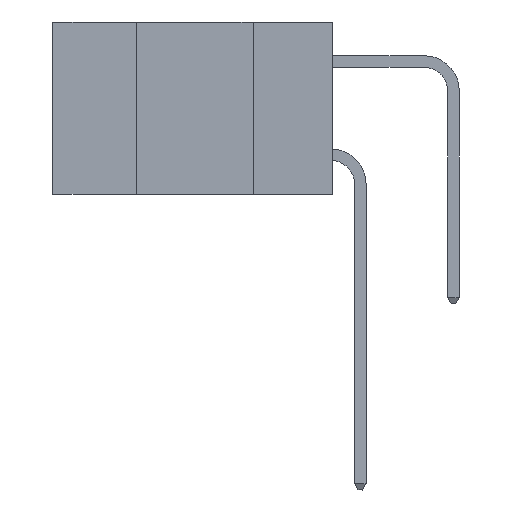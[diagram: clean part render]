
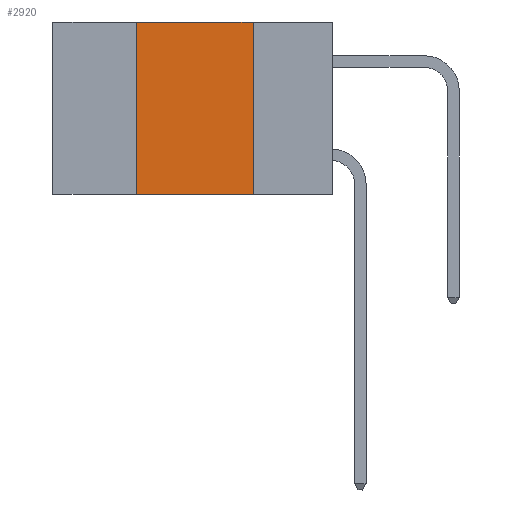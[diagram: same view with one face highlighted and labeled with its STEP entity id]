
A CAD part, left-side view. The second image highlights one B-rep face of the part: STEP entity #2920.
In plain terms, the highlighted planar face has unit normal (-1, 0, 0).
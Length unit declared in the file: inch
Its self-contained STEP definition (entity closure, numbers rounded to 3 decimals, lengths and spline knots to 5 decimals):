
#825 = EDGE_CURVE ( 'NONE', #7710, #1004, #13424, .T. ) ;
#835 = DIRECTION ( 'NONE',  ( 0., -1., 0. ) ) ;
#1004 = VERTEX_POINT ( 'NONE', #12930 ) ;
#1576 = VERTEX_POINT ( 'NONE', #9595 ) ;
#1838 = EDGE_LOOP ( 'NONE', ( #1877, #1987, #2013, #2182 ) ) ;
#1877 = ORIENTED_EDGE ( 'NONE', *, *, #9622, .F. ) ;
#1918 = VECTOR ( 'NONE', #5620, 39.37008 ) ;
#1955 = VERTEX_POINT ( 'NONE', #13369 ) ;
#1987 = ORIENTED_EDGE ( 'NONE', *, *, #13749, .F. ) ;
#2013 = ORIENTED_EDGE ( 'NONE', *, *, #4867, .F. ) ;
#2172 = FACE_OUTER_BOUND ( 'NONE', #1838, .T. ) ;
#2182 = ORIENTED_EDGE ( 'NONE', *, *, #825, .T. ) ;
#2338 = CARTESIAN_POINT ( 'NONE',  ( 0., 0.6, 0. ) ) ;
#2412 = LINE ( 'NONE', #2338, #13441 ) ;
#2836 = CARTESIAN_POINT ( 'NONE',  ( 0., 0.42, -0.37 ) ) ;
#2920 = ADVANCED_FACE ( 'NONE', ( #2172 ), #12034, .F. ) ;
#4664 = DIRECTION ( 'NONE',  ( 0., -1., 0. ) ) ;
#4845 = CARTESIAN_POINT ( 'NONE',  ( 0., 0.42, 0. ) ) ;
#4867 = EDGE_CURVE ( 'NONE', #7710, #1955, #12949, .T. ) ;
#5620 = DIRECTION ( 'NONE',  ( 0., 0., 1. ) ) ;
#5659 = CARTESIAN_POINT ( 'NONE',  ( 0., 0.6, -0.37 ) ) ;
#6917 = AXIS2_PLACEMENT_3D ( 'NONE', #8811, #9266, #10888 ) ;
#7131 = CARTESIAN_POINT ( 'NONE',  ( 0., 0.17, 0. ) ) ;
#7147 = VECTOR ( 'NONE', #8162, 39.37008 ) ;
#7710 = VERTEX_POINT ( 'NONE', #2836 ) ;
#8162 = DIRECTION ( 'NONE',  ( 0., 0., -1. ) ) ;
#8811 = CARTESIAN_POINT ( 'NONE',  ( 0., 0.6, 0. ) ) ;
#9266 = DIRECTION ( 'NONE',  ( 1., 0., 0. ) ) ;
#9595 = CARTESIAN_POINT ( 'NONE',  ( 0., 0.17, 0. ) ) ;
#9622 = EDGE_CURVE ( 'NONE', #1576, #1004, #9872, .T. ) ;
#9872 = LINE ( 'NONE', #7131, #7147 ) ;
#10621 = VECTOR ( 'NONE', #835, 39.37008 ) ;
#10888 = DIRECTION ( 'NONE',  ( 0., 0., -1. ) ) ;
#12034 = PLANE ( 'NONE',  #6917 ) ;
#12930 = CARTESIAN_POINT ( 'NONE',  ( 0., 0.17, -0.37 ) ) ;
#12949 = LINE ( 'NONE', #4845, #1918 ) ;
#13369 = CARTESIAN_POINT ( 'NONE',  ( 0., 0.42, 0. ) ) ;
#13424 = LINE ( 'NONE', #5659, #10621 ) ;
#13441 = VECTOR ( 'NONE', #4664, 39.37008 ) ;
#13749 = EDGE_CURVE ( 'NONE', #1955, #1576, #2412, .T. ) ;
